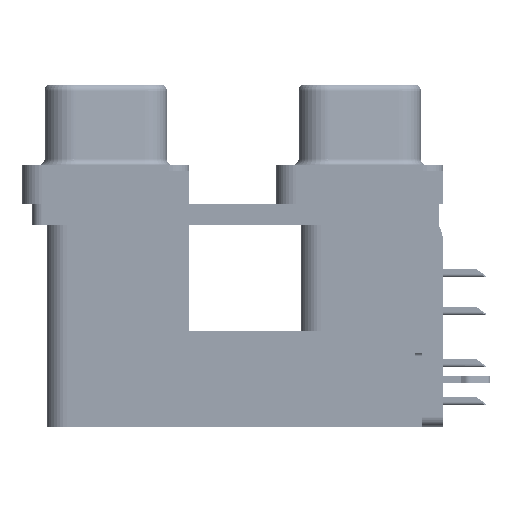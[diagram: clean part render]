
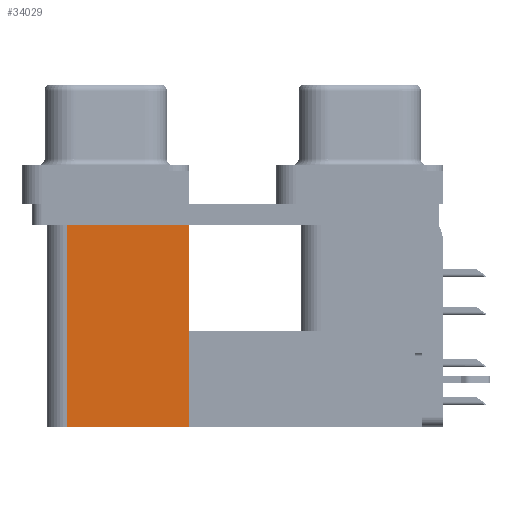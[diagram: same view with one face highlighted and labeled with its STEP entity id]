
A CAD part, left-side view. The second image highlights one B-rep face of the part: STEP entity #34029.
In plain terms, the highlighted planar face has unit normal (-1, 0, 0).
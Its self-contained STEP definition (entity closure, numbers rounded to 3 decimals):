
#1053 = VECTOR ( 'NONE', #10930, 1000. ) ;
#5058 = EDGE_CURVE ( 'NONE', #24254, #49214, #34788, .T. ) ;
#6568 = ORIENTED_EDGE ( 'NONE', *, *, #32341, .F. ) ;
#7396 = DIRECTION ( 'NONE',  ( 0., 0., 1. ) ) ;
#9755 = CARTESIAN_POINT ( 'NONE',  ( 3.79, 12.775, -2.5 ) ) ;
#10930 = DIRECTION ( 'NONE',  ( 0., 1., 0. ) ) ;
#11654 = LINE ( 'NONE', #33155, #27957 ) ;
#17125 = CARTESIAN_POINT ( 'NONE',  ( 3.79, 12.775, -19.2 ) ) ;
#18147 = VERTEX_POINT ( 'NONE', #25139 ) ;
#18175 = VECTOR ( 'NONE', #46802, 1000. ) ;
#18309 = CARTESIAN_POINT ( 'NONE',  ( 3.79, 21.975, -19.2 ) ) ;
#19434 = CARTESIAN_POINT ( 'NONE',  ( 3.79, 12.775, -2.5 ) ) ;
#19991 = EDGE_CURVE ( 'NONE', #18147, #50852, #35168, .T. ) ;
#21642 = DIRECTION ( 'NONE',  ( 1., 0., 0. ) ) ;
#22176 = FACE_OUTER_BOUND ( 'NONE', #38692, .T. ) ;
#22618 = CARTESIAN_POINT ( 'NONE',  ( 3.79, 21.975, -2.5 ) ) ;
#22670 = CARTESIAN_POINT ( 'NONE',  ( 3.79, 12.775, -19.2 ) ) ;
#24254 = VERTEX_POINT ( 'NONE', #19434 ) ;
#25139 = CARTESIAN_POINT ( 'NONE',  ( 3.79, 12.775, -19.2 ) ) ;
#26722 = ORIENTED_EDGE ( 'NONE', *, *, #19991, .F. ) ;
#27957 = VECTOR ( 'NONE', #7396, 1000. ) ;
#32341 = EDGE_CURVE ( 'NONE', #50852, #49214, #41344, .T. ) ;
#33155 = CARTESIAN_POINT ( 'NONE',  ( 3.79, 12.775, -19.2 ) ) ;
#33350 = AXIS2_PLACEMENT_3D ( 'NONE', #17125, #21642, #50429 ) ;
#33356 = VECTOR ( 'NONE', #33842, 1000. ) ;
#33578 = CARTESIAN_POINT ( 'NONE',  ( 3.79, 21.975, -19.2 ) ) ;
#33842 = DIRECTION ( 'NONE',  ( 0., 0., 1. ) ) ;
#34029 = ADVANCED_FACE ( 'NONE', ( #22176 ), #41415, .F. ) ;
#34788 = LINE ( 'NONE', #9755, #18175 ) ;
#35168 = LINE ( 'NONE', #22670, #1053 ) ;
#37958 = ORIENTED_EDGE ( 'NONE', *, *, #5058, .T. ) ;
#38692 = EDGE_LOOP ( 'NONE', ( #37958, #6568, #26722, #42161 ) ) ;
#41344 = LINE ( 'NONE', #33578, #33356 ) ;
#41415 = PLANE ( 'NONE',  #33350 ) ;
#42161 = ORIENTED_EDGE ( 'NONE', *, *, #46511, .T. ) ;
#46511 = EDGE_CURVE ( 'NONE', #18147, #24254, #11654, .T. ) ;
#46802 = DIRECTION ( 'NONE',  ( 0., 1., 0. ) ) ;
#49214 = VERTEX_POINT ( 'NONE', #22618 ) ;
#50429 = DIRECTION ( 'NONE',  ( 0., 0., -1. ) ) ;
#50852 = VERTEX_POINT ( 'NONE', #18309 ) ;
